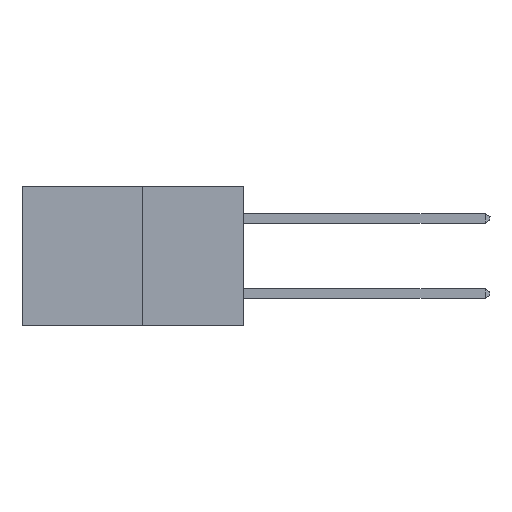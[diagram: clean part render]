
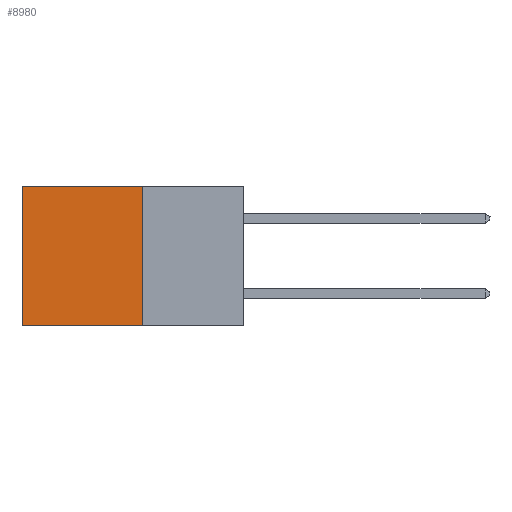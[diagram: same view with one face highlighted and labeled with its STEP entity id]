
A CAD part, left-side view. The second image highlights one B-rep face of the part: STEP entity #8980.
In plain terms, the highlighted planar face has unit normal (-1, 0, 0).
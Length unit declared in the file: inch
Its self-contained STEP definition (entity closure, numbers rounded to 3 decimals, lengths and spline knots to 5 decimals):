
#481 = ORIENTED_EDGE ( 'NONE', *, *, #12737, .F. ) ;
#763 = DIRECTION ( 'NONE',  ( 0., 1., 0. ) ) ;
#881 = DIRECTION ( 'NONE',  ( 0., 0., -1. ) ) ;
#934 = VECTOR ( 'NONE', #763, 39.37008 ) ;
#1102 = EDGE_CURVE ( 'NONE', #10490, #16524, #21452, .T. ) ;
#1195 = CARTESIAN_POINT ( 'NONE',  ( 0.277, 0.27, 0. ) ) ;
#1532 = LINE ( 'NONE', #1195, #934 ) ;
#3561 = VERTEX_POINT ( 'NONE', #12252 ) ;
#4270 = VECTOR ( 'NONE', #5485, 39.37008 ) ;
#5485 = DIRECTION ( 'NONE',  ( 0., 0., -1. ) ) ;
#5646 = FACE_OUTER_BOUND ( 'NONE', #8569, .T. ) ;
#6062 = VECTOR ( 'NONE', #7421, 39.37008 ) ;
#6340 = CARTESIAN_POINT ( 'NONE',  ( 0.277, 0.59, 0. ) ) ;
#6419 = EDGE_CURVE ( 'NONE', #3561, #14809, #1532, .T. ) ;
#7421 = DIRECTION ( 'NONE',  ( 0., 1., 0. ) ) ;
#8046 = CARTESIAN_POINT ( 'NONE',  ( 0.277, 0.27, -0.37 ) ) ;
#8569 = EDGE_LOOP ( 'NONE', ( #13579, #19256, #481, #17175 ) ) ;
#8980 = ADVANCED_FACE ( 'NONE', ( #5646 ), #23960, .F. ) ;
#9478 = CARTESIAN_POINT ( 'NONE',  ( 0.277, 0.59, -0.37 ) ) ;
#10392 = CARTESIAN_POINT ( 'NONE',  ( 0.277, 0.59, -0.37 ) ) ;
#10490 = VERTEX_POINT ( 'NONE', #22428 ) ;
#12252 = CARTESIAN_POINT ( 'NONE',  ( 0.277, 0.27, 0. ) ) ;
#12547 = DIRECTION ( 'NONE',  ( 1., 0., 0. ) ) ;
#12737 = EDGE_CURVE ( 'NONE', #3561, #10490, #18647, .T. ) ;
#13579 = ORIENTED_EDGE ( 'NONE', *, *, #14524, .T. ) ;
#14160 = VECTOR ( 'NONE', #21508, 39.37008 ) ;
#14524 = EDGE_CURVE ( 'NONE', #14809, #16524, #24161, .T. ) ;
#14809 = VERTEX_POINT ( 'NONE', #6340 ) ;
#16524 = VERTEX_POINT ( 'NONE', #10392 ) ;
#17175 = ORIENTED_EDGE ( 'NONE', *, *, #6419, .T. ) ;
#18647 = LINE ( 'NONE', #8046, #14160 ) ;
#19256 = ORIENTED_EDGE ( 'NONE', *, *, #1102, .F. ) ;
#20167 = CARTESIAN_POINT ( 'NONE',  ( 0.277, 0.27, -0.37 ) ) ;
#20293 = AXIS2_PLACEMENT_3D ( 'NONE', #20167, #12547, #881 ) ;
#21452 = LINE ( 'NONE', #22218, #6062 ) ;
#21508 = DIRECTION ( 'NONE',  ( 0., 0., -1. ) ) ;
#22218 = CARTESIAN_POINT ( 'NONE',  ( 0.277, 0.27, -0.37 ) ) ;
#22428 = CARTESIAN_POINT ( 'NONE',  ( 0.277, 0.27, -0.37 ) ) ;
#23960 = PLANE ( 'NONE',  #20293 ) ;
#24161 = LINE ( 'NONE', #9478, #4270 ) ;
